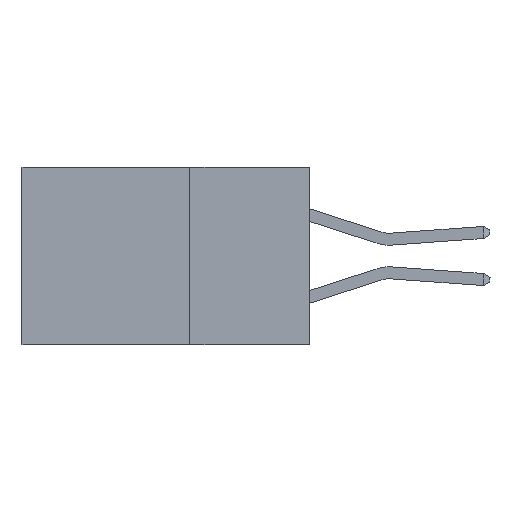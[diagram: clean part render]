
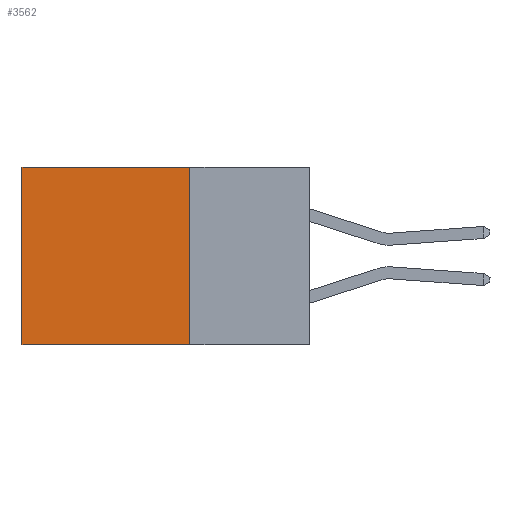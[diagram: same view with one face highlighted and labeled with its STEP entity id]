
A CAD part, left-side view. The second image highlights one B-rep face of the part: STEP entity #3562.
In plain terms, the highlighted planar face has unit normal (-1, 0, 0).
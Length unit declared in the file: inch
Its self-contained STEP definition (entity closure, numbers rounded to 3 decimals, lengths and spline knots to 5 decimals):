
#642 = CARTESIAN_POINT ( 'NONE',  ( 0.2615, 0.25, 0. ) ) ;
#884 = VERTEX_POINT ( 'NONE', #10189 ) ;
#1898 = CARTESIAN_POINT ( 'NONE',  ( 0.2615, 0.25, -0.37 ) ) ;
#2536 = AXIS2_PLACEMENT_3D ( 'NONE', #16314, #17025, #16927 ) ;
#2537 = DIRECTION ( 'NONE',  ( 0., 1., 0. ) ) ;
#2597 = VECTOR ( 'NONE', #2537, 39.37008 ) ;
#2798 = FACE_OUTER_BOUND ( 'NONE', #12696, .T. ) ;
#3026 = DIRECTION ( 'NONE',  ( 0., 0., -1. ) ) ;
#3503 = EDGE_CURVE ( 'NONE', #8478, #6209, #14235, .T. ) ;
#3562 = ADVANCED_FACE ( 'NONE', ( #2798 ), #11287, .F. ) ;
#3619 = EDGE_CURVE ( 'NONE', #6209, #9579, #6813, .T. ) ;
#3681 = VECTOR ( 'NONE', #6409, 39.37008 ) ;
#3811 = EDGE_CURVE ( 'NONE', #884, #9579, #6614, .T. ) ;
#4036 = LINE ( 'NONE', #17178, #14620 ) ;
#4527 = CARTESIAN_POINT ( 'NONE',  ( 0.2615, 0.6, -0.37 ) ) ;
#4833 = EDGE_CURVE ( 'NONE', #8478, #884, #4036, .T. ) ;
#6209 = VERTEX_POINT ( 'NONE', #8092 ) ;
#6409 = DIRECTION ( 'NONE',  ( 0., 1., 0. ) ) ;
#6614 = LINE ( 'NONE', #1898, #2597 ) ;
#6813 = LINE ( 'NONE', #16342, #12530 ) ;
#7933 = CARTESIAN_POINT ( 'NONE',  ( 0.2615, 0.25, 0. ) ) ;
#8092 = CARTESIAN_POINT ( 'NONE',  ( 0.2615, 0.6, 0. ) ) ;
#8478 = VERTEX_POINT ( 'NONE', #642 ) ;
#9579 = VERTEX_POINT ( 'NONE', #4527 ) ;
#10189 = CARTESIAN_POINT ( 'NONE',  ( 0.2615, 0.25, -0.37 ) ) ;
#11287 = PLANE ( 'NONE',  #2536 ) ;
#12148 = ORIENTED_EDGE ( 'NONE', *, *, #3503, .T. ) ;
#12355 = ORIENTED_EDGE ( 'NONE', *, *, #3811, .F. ) ;
#12530 = VECTOR ( 'NONE', #15300, 39.37008 ) ;
#12696 = EDGE_LOOP ( 'NONE', ( #12832, #12355, #14067, #12148 ) ) ;
#12832 = ORIENTED_EDGE ( 'NONE', *, *, #3619, .T. ) ;
#14067 = ORIENTED_EDGE ( 'NONE', *, *, #4833, .F. ) ;
#14235 = LINE ( 'NONE', #7933, #3681 ) ;
#14620 = VECTOR ( 'NONE', #3026, 39.37008 ) ;
#15300 = DIRECTION ( 'NONE',  ( 0., 0., -1. ) ) ;
#16314 = CARTESIAN_POINT ( 'NONE',  ( 0.2615, 0.25, -0.37 ) ) ;
#16342 = CARTESIAN_POINT ( 'NONE',  ( 0.2615, 0.6, -0.37 ) ) ;
#16927 = DIRECTION ( 'NONE',  ( 0., 0., -1. ) ) ;
#17025 = DIRECTION ( 'NONE',  ( 1., 0., 0. ) ) ;
#17178 = CARTESIAN_POINT ( 'NONE',  ( 0.2615, 0.25, -0.37 ) ) ;
